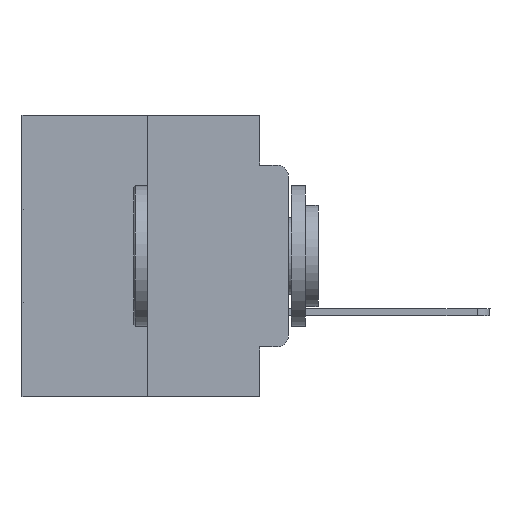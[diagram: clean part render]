
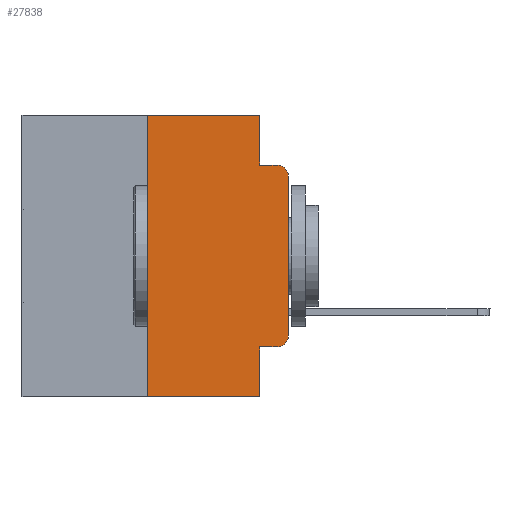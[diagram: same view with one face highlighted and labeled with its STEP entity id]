
A CAD part, left-side view. The second image highlights one B-rep face of the part: STEP entity #27838.
In plain terms, the highlighted planar face has unit normal (-1, 0, 0).
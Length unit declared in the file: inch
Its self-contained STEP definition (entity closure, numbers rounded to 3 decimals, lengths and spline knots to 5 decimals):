
#130 = CARTESIAN_POINT ( 'NONE',  ( 0., 0.051, -0.5 ) ) ;
#993 = CARTESIAN_POINT ( 'NONE',  ( 0., 0.051, 0. ) ) ;
#1058 = DIRECTION ( 'NONE',  ( 0., 0., -1. ) ) ;
#1129 = PLANE ( 'NONE',  #10913 ) ;
#1140 = CARTESIAN_POINT ( 'NONE',  ( 0., 0.25, 0. ) ) ;
#1155 = CIRCLE ( 'NONE', #17117, 0.02 ) ;
#1324 = CARTESIAN_POINT ( 'NONE',  ( 0., 0.473, 0. ) ) ;
#1464 = VECTOR ( 'NONE', #15470, 39.37008 ) ;
#2110 = EDGE_CURVE ( 'NONE', #19455, #10753, #4717, .T. ) ;
#2517 = EDGE_CURVE ( 'NONE', #9466, #10753, #15838, .T. ) ;
#3208 = DIRECTION ( 'NONE',  ( 0., -1., 0. ) ) ;
#4087 = CARTESIAN_POINT ( 'NONE',  ( 0., 0., -0.3915 ) ) ;
#4565 = VECTOR ( 'NONE', #15876, 39.37008 ) ;
#4596 = CIRCLE ( 'NONE', #22829, 0.02 ) ;
#4717 = LINE ( 'NONE', #993, #4565 ) ;
#5220 = VECTOR ( 'NONE', #16053, 39.37008 ) ;
#5287 = DIRECTION ( 'NONE',  ( 1., 0., 0. ) ) ;
#6150 = VERTEX_POINT ( 'NONE', #10477 ) ;
#6528 = VERTEX_POINT ( 'NONE', #18426 ) ;
#6844 = DIRECTION ( 'NONE',  ( 0., -1., 0. ) ) ;
#7022 = LINE ( 'NONE', #1140, #10821 ) ;
#7127 = VERTEX_POINT ( 'NONE', #15647 ) ;
#7261 = CARTESIAN_POINT ( 'NONE',  ( 0., 0.473, -0.5 ) ) ;
#7519 = EDGE_CURVE ( 'NONE', #19911, #7127, #18153, .T. ) ;
#8246 = ORIENTED_EDGE ( 'NONE', *, *, #9306, .F. ) ;
#8489 = VECTOR ( 'NONE', #27169, 39.37008 ) ;
#9223 = LINE ( 'NONE', #20627, #11758 ) ;
#9306 = EDGE_CURVE ( 'NONE', #9466, #6150, #7022, .T. ) ;
#9466 = VERTEX_POINT ( 'NONE', #14288 ) ;
#9495 = CARTESIAN_POINT ( 'NONE',  ( 0., 0.02, -0.0885 ) ) ;
#10441 = ORIENTED_EDGE ( 'NONE', *, *, #21444, .F. ) ;
#10477 = CARTESIAN_POINT ( 'NONE',  ( 0., 0.25, 0. ) ) ;
#10753 = VERTEX_POINT ( 'NONE', #130 ) ;
#10821 = VECTOR ( 'NONE', #18269, 39.37008 ) ;
#10913 = AXIS2_PLACEMENT_3D ( 'NONE', #27280, #5287, #11723 ) ;
#11008 = DIRECTION ( 'NONE',  ( -1., 0., 0. ) ) ;
#11468 = CARTESIAN_POINT ( 'NONE',  ( 0., 0.02, -0.3915 ) ) ;
#11606 = ORIENTED_EDGE ( 'NONE', *, *, #26452, .F. ) ;
#11646 = CARTESIAN_POINT ( 'NONE',  ( 0., 0.02, -0.1085 ) ) ;
#11723 = DIRECTION ( 'NONE',  ( 0., 0., -1. ) ) ;
#11758 = VECTOR ( 'NONE', #11936, 39.37008 ) ;
#11808 = LINE ( 'NONE', #20780, #13400 ) ;
#11936 = DIRECTION ( 'NONE',  ( 0., 0., -1. ) ) ;
#13400 = VECTOR ( 'NONE', #3208, 39.37008 ) ;
#14144 = FACE_OUTER_BOUND ( 'NONE', #22578, .T. ) ;
#14288 = CARTESIAN_POINT ( 'NONE',  ( 0., 0.25, -0.5 ) ) ;
#14952 = EDGE_CURVE ( 'NONE', #7127, #24130, #4596, .T. ) ;
#15119 = VECTOR ( 'NONE', #6844, 39.37008 ) ;
#15191 = CARTESIAN_POINT ( 'NONE',  ( 0., 0.051, -0.4115 ) ) ;
#15222 = VERTEX_POINT ( 'NONE', #26608 ) ;
#15470 = DIRECTION ( 'NONE',  ( 0., -1., 0. ) ) ;
#15647 = CARTESIAN_POINT ( 'NONE',  ( 0., 0., -0.1085 ) ) ;
#15838 = LINE ( 'NONE', #7261, #15119 ) ;
#15876 = DIRECTION ( 'NONE',  ( 0., 0., -1. ) ) ;
#15905 = CARTESIAN_POINT ( 'NONE',  ( 0., 0., 0. ) ) ;
#16053 = DIRECTION ( 'NONE',  ( 0., -1., 0. ) ) ;
#16212 = DIRECTION ( 'NONE',  ( -1., 0., 0. ) ) ;
#16399 = VERTEX_POINT ( 'NONE', #23878 ) ;
#17117 = AXIS2_PLACEMENT_3D ( 'NONE', #11468, #11008, #23400 ) ;
#17569 = ORIENTED_EDGE ( 'NONE', *, *, #7519, .T. ) ;
#18081 = ORIENTED_EDGE ( 'NONE', *, *, #2517, .T. ) ;
#18153 = LINE ( 'NONE', #15905, #8489 ) ;
#18269 = DIRECTION ( 'NONE',  ( 0., 0., 1. ) ) ;
#18279 = EDGE_CURVE ( 'NONE', #19455, #16399, #20407, .T. ) ;
#18426 = CARTESIAN_POINT ( 'NONE',  ( 0., 0.051, 0. ) ) ;
#19455 = VERTEX_POINT ( 'NONE', #22704 ) ;
#19701 = ORIENTED_EDGE ( 'NONE', *, *, #2110, .F. ) ;
#19911 = VERTEX_POINT ( 'NONE', #4087 ) ;
#20407 = LINE ( 'NONE', #15191, #1464 ) ;
#20627 = CARTESIAN_POINT ( 'NONE',  ( 0., 0.051, 0. ) ) ;
#20780 = CARTESIAN_POINT ( 'NONE',  ( 0., 0.051, -0.0885 ) ) ;
#20891 = LINE ( 'NONE', #1324, #5220 ) ;
#21444 = EDGE_CURVE ( 'NONE', #15222, #24130, #11808, .T. ) ;
#21933 = EDGE_CURVE ( 'NONE', #6150, #6528, #20891, .T. ) ;
#22093 = ORIENTED_EDGE ( 'NONE', *, *, #18279, .T. ) ;
#22142 = ORIENTED_EDGE ( 'NONE', *, *, #14952, .T. ) ;
#22324 = ORIENTED_EDGE ( 'NONE', *, *, #21933, .F. ) ;
#22578 = EDGE_LOOP ( 'NONE', ( #17569, #22142, #10441, #11606, #22324, #8246, #18081, #19701, #22093, #25034 ) ) ;
#22704 = CARTESIAN_POINT ( 'NONE',  ( 0., 0.051, -0.4115 ) ) ;
#22829 = AXIS2_PLACEMENT_3D ( 'NONE', #11646, #16212, #1058 ) ;
#23400 = DIRECTION ( 'NONE',  ( 0., 0., -1. ) ) ;
#23444 = EDGE_CURVE ( 'NONE', #16399, #19911, #1155, .T. ) ;
#23878 = CARTESIAN_POINT ( 'NONE',  ( 0., 0.02, -0.4115 ) ) ;
#24130 = VERTEX_POINT ( 'NONE', #9495 ) ;
#25034 = ORIENTED_EDGE ( 'NONE', *, *, #23444, .T. ) ;
#26452 = EDGE_CURVE ( 'NONE', #6528, #15222, #9223, .T. ) ;
#26608 = CARTESIAN_POINT ( 'NONE',  ( 0., 0.051, -0.0885 ) ) ;
#27169 = DIRECTION ( 'NONE',  ( 0., 0., 1. ) ) ;
#27280 = CARTESIAN_POINT ( 'NONE',  ( 0., 0.473, 0. ) ) ;
#27838 = ADVANCED_FACE ( 'NONE', ( #14144 ), #1129, .F. ) ;
